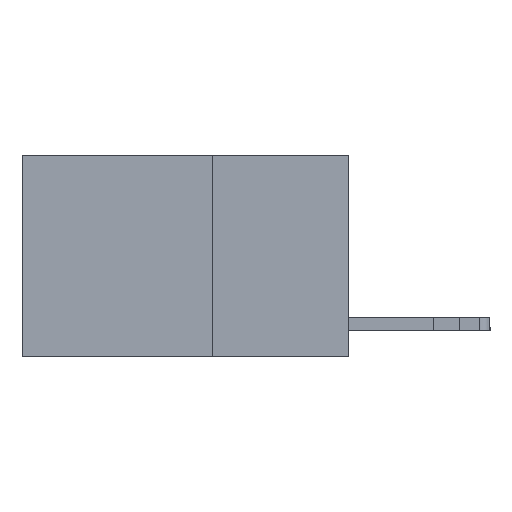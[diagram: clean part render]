
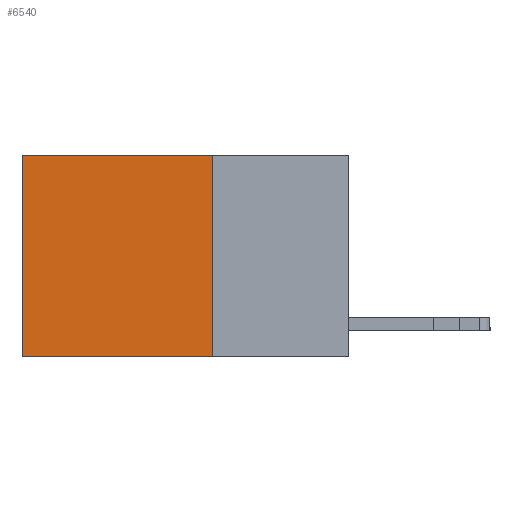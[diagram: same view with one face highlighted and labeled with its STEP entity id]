
A CAD part, left-side view. The second image highlights one B-rep face of the part: STEP entity #6540.
In plain terms, the highlighted planar face has unit normal (-1, 0, 0).
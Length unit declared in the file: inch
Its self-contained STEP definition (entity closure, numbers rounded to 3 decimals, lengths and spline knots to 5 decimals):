
#34 = EDGE_LOOP ( 'NONE', ( #6571, #1145, #5121, #710 ) ) ;
#372 = VERTEX_POINT ( 'NONE', #7080 ) ;
#489 = DIRECTION ( 'NONE',  ( 0., 0., -1. ) ) ;
#564 = CARTESIAN_POINT ( 'NONE',  ( 0.2625, 0.25, 0. ) ) ;
#710 = ORIENTED_EDGE ( 'NONE', *, *, #12077, .T. ) ;
#1145 = ORIENTED_EDGE ( 'NONE', *, *, #4342, .F. ) ;
#1331 = LINE ( 'NONE', #11753, #8779 ) ;
#1555 = DIRECTION ( 'NONE',  ( 1., 0., 0. ) ) ;
#1830 = CARTESIAN_POINT ( 'NONE',  ( 0.2625, 0.25, 0. ) ) ;
#2400 = DIRECTION ( 'NONE',  ( 0., 1., 0. ) ) ;
#3134 = VERTEX_POINT ( 'NONE', #6181 ) ;
#3344 = LINE ( 'NONE', #7157, #6017 ) ;
#3451 = CARTESIAN_POINT ( 'NONE',  ( 0.2625, 0.25, 0. ) ) ;
#3517 = FACE_OUTER_BOUND ( 'NONE', #34, .T. ) ;
#3818 = AXIS2_PLACEMENT_3D ( 'NONE', #3451, #1555, #489 ) ;
#4342 = EDGE_CURVE ( 'NONE', #5342, #3134, #7715, .T. ) ;
#4662 = EDGE_CURVE ( 'NONE', #12248, #5342, #5458, .T. ) ;
#5121 = ORIENTED_EDGE ( 'NONE', *, *, #4662, .F. ) ;
#5342 = VERTEX_POINT ( 'NONE', #10940 ) ;
#5458 = LINE ( 'NONE', #564, #8357 ) ;
#5507 = PLANE ( 'NONE',  #3818 ) ;
#6017 = VECTOR ( 'NONE', #11296, 39.37008 ) ;
#6181 = CARTESIAN_POINT ( 'NONE',  ( 0.2625, 0.6, -0.37 ) ) ;
#6540 = ADVANCED_FACE ( 'NONE', ( #3517 ), #5507, .F. ) ;
#6571 = ORIENTED_EDGE ( 'NONE', *, *, #7429, .T. ) ;
#7080 = CARTESIAN_POINT ( 'NONE',  ( 0.2625, 0.6, 0. ) ) ;
#7157 = CARTESIAN_POINT ( 'NONE',  ( 0.2625, 0.6, 0. ) ) ;
#7429 = EDGE_CURVE ( 'NONE', #372, #3134, #3344, .T. ) ;
#7715 = LINE ( 'NONE', #7831, #9747 ) ;
#7831 = CARTESIAN_POINT ( 'NONE',  ( 0.2625, 0.25, -0.37 ) ) ;
#8206 = DIRECTION ( 'NONE',  ( 0., 0., -1. ) ) ;
#8357 = VECTOR ( 'NONE', #8206, 39.37008 ) ;
#8779 = VECTOR ( 'NONE', #2400, 39.37008 ) ;
#8900 = DIRECTION ( 'NONE',  ( 0., 1., 0. ) ) ;
#9747 = VECTOR ( 'NONE', #8900, 39.37008 ) ;
#10940 = CARTESIAN_POINT ( 'NONE',  ( 0.2625, 0.25, -0.37 ) ) ;
#11296 = DIRECTION ( 'NONE',  ( 0., 0., -1. ) ) ;
#11753 = CARTESIAN_POINT ( 'NONE',  ( 0.2625, 0.25, 0. ) ) ;
#12077 = EDGE_CURVE ( 'NONE', #12248, #372, #1331, .T. ) ;
#12248 = VERTEX_POINT ( 'NONE', #1830 ) ;
